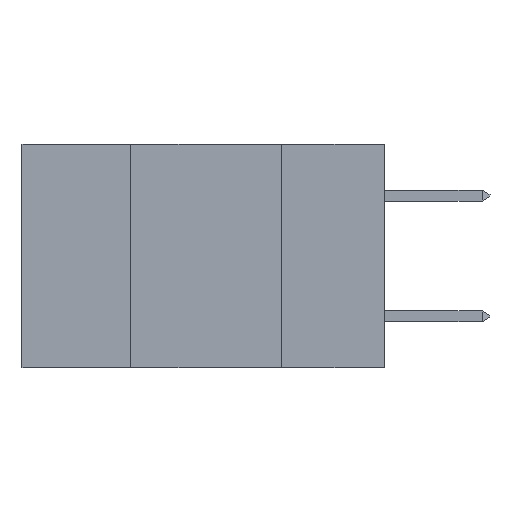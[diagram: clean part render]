
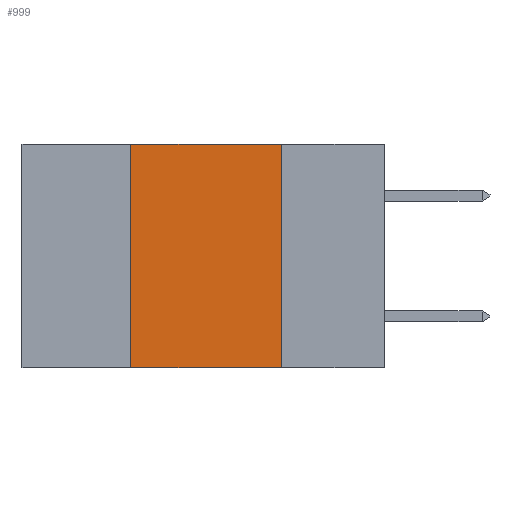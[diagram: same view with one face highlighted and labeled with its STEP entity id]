
A CAD part, left-side view. The second image highlights one B-rep face of the part: STEP entity #999.
In plain terms, the highlighted planar face has unit normal (-1, 0, 0).
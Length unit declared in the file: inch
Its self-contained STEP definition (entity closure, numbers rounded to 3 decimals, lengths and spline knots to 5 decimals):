
#260 = ORIENTED_EDGE ( 'NONE', *, *, #12431, .F. ) ;
#817 = DIRECTION ( 'NONE',  ( 0., 0., -1. ) ) ;
#999 = ADVANCED_FACE ( 'NONE', ( #2847 ), #12583, .F. ) ;
#1345 = DIRECTION ( 'NONE',  ( 1., 0., 0. ) ) ;
#2187 = LINE ( 'NONE', #4057, #12047 ) ;
#2285 = VERTEX_POINT ( 'NONE', #4091 ) ;
#2728 = VERTEX_POINT ( 'NONE', #4210 ) ;
#2847 = FACE_OUTER_BOUND ( 'NONE', #14668, .T. ) ;
#3518 = CARTESIAN_POINT ( 'NONE',  ( 0., 0.17, 0. ) ) ;
#3705 = ORIENTED_EDGE ( 'NONE', *, *, #4895, .F. ) ;
#3963 = DIRECTION ( 'NONE',  ( 0., -1., 0. ) ) ;
#4057 = CARTESIAN_POINT ( 'NONE',  ( 0., 0.42, 0. ) ) ;
#4091 = CARTESIAN_POINT ( 'NONE',  ( 0., 0.17, -0.37 ) ) ;
#4210 = CARTESIAN_POINT ( 'NONE',  ( 0., 0.17, 0. ) ) ;
#4857 = VECTOR ( 'NONE', #817, 39.37008 ) ;
#4895 = EDGE_CURVE ( 'NONE', #6460, #2728, #10301, .T. ) ;
#6460 = VERTEX_POINT ( 'NONE', #11965 ) ;
#6569 = CARTESIAN_POINT ( 'NONE',  ( 0., 0.6, 0. ) ) ;
#7608 = DIRECTION ( 'NONE',  ( 0., -1., 0. ) ) ;
#7634 = LINE ( 'NONE', #3518, #4857 ) ;
#7732 = AXIS2_PLACEMENT_3D ( 'NONE', #15129, #1345, #15018 ) ;
#7757 = EDGE_CURVE ( 'NONE', #2728, #2285, #7634, .T. ) ;
#7886 = DIRECTION ( 'NONE',  ( 0., 0., 1. ) ) ;
#9099 = VECTOR ( 'NONE', #7608, 39.37008 ) ;
#10301 = LINE ( 'NONE', #6569, #13245 ) ;
#11319 = CARTESIAN_POINT ( 'NONE',  ( 0., 0.42, -0.37 ) ) ;
#11898 = EDGE_CURVE ( 'NONE', #13850, #2285, #15984, .T. ) ;
#11965 = CARTESIAN_POINT ( 'NONE',  ( 0., 0.42, 0. ) ) ;
#12047 = VECTOR ( 'NONE', #7886, 39.37008 ) ;
#12431 = EDGE_CURVE ( 'NONE', #13850, #6460, #2187, .T. ) ;
#12583 = PLANE ( 'NONE',  #7732 ) ;
#12603 = CARTESIAN_POINT ( 'NONE',  ( 0., 0.6, -0.37 ) ) ;
#12990 = ORIENTED_EDGE ( 'NONE', *, *, #11898, .T. ) ;
#13245 = VECTOR ( 'NONE', #3963, 39.37008 ) ;
#13850 = VERTEX_POINT ( 'NONE', #11319 ) ;
#14668 = EDGE_LOOP ( 'NONE', ( #15591, #3705, #260, #12990 ) ) ;
#15018 = DIRECTION ( 'NONE',  ( 0., 0., -1. ) ) ;
#15129 = CARTESIAN_POINT ( 'NONE',  ( 0., 0.6, 0. ) ) ;
#15591 = ORIENTED_EDGE ( 'NONE', *, *, #7757, .F. ) ;
#15984 = LINE ( 'NONE', #12603, #9099 ) ;
